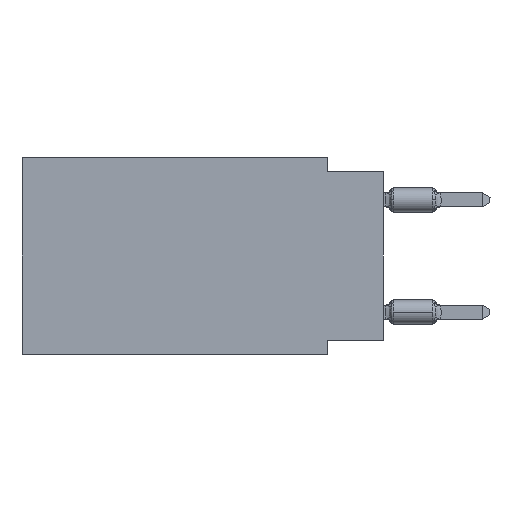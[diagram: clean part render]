
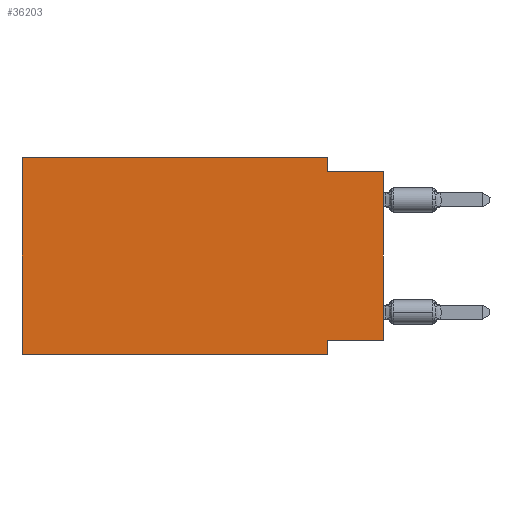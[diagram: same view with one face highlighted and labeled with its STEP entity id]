
A CAD part, left-side view. The second image highlights one B-rep face of the part: STEP entity #36203.
In plain terms, the highlighted planar face has unit normal (-1, 0, 0).
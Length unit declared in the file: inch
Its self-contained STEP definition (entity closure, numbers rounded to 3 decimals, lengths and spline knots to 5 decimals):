
#1443 = VERTEX_POINT ( 'NONE', #53261 ) ;
#1887 = ORIENTED_EDGE ( 'NONE', *, *, #59351, .F. ) ;
#2202 = CARTESIAN_POINT ( 'NONE',  ( 0., 0.645, -0.35 ) ) ;
#2597 = CARTESIAN_POINT ( 'NONE',  ( 0., 0., 0. ) ) ;
#3187 = VECTOR ( 'NONE', #30188, 39.37008 ) ;
#3581 = ORIENTED_EDGE ( 'NONE', *, *, #48791, .F. ) ;
#4973 = DIRECTION ( 'NONE',  ( 0., 0., 1. ) ) ;
#5884 = LINE ( 'NONE', #10403, #34656 ) ;
#6869 = CARTESIAN_POINT ( 'NONE',  ( 0., 0.645, 0. ) ) ;
#6891 = VECTOR ( 'NONE', #37320, 39.37008 ) ;
#8120 = VECTOR ( 'NONE', #14728, 39.37008 ) ;
#9150 = EDGE_CURVE ( 'NONE', #45152, #1443, #17532, .T. ) ;
#9815 = VECTOR ( 'NONE', #4973, 39.37008 ) ;
#10074 = CARTESIAN_POINT ( 'NONE',  ( 0., 0.1, -0.025 ) ) ;
#10147 = CARTESIAN_POINT ( 'NONE',  ( 0., 0.645, 0. ) ) ;
#10403 = CARTESIAN_POINT ( 'NONE',  ( 0., 0.645, -0.35 ) ) ;
#11067 = EDGE_CURVE ( 'NONE', #25647, #43677, #47389, .T. ) ;
#11736 = PLANE ( 'NONE',  #49026 ) ;
#14728 = DIRECTION ( 'NONE',  ( 0., 0., -1. ) ) ;
#15031 = LINE ( 'NONE', #10147, #9815 ) ;
#16442 = CARTESIAN_POINT ( 'NONE',  ( 0., 0., -0.325 ) ) ;
#17162 = VECTOR ( 'NONE', #35926, 39.37008 ) ;
#17532 = LINE ( 'NONE', #51068, #25359 ) ;
#22454 = ORIENTED_EDGE ( 'NONE', *, *, #25633, .F. ) ;
#22776 = ORIENTED_EDGE ( 'NONE', *, *, #9150, .F. ) ;
#24772 = CARTESIAN_POINT ( 'NONE',  ( 0., 0., -0.325 ) ) ;
#25254 = CARTESIAN_POINT ( 'NONE',  ( 0., 0., -0.025 ) ) ;
#25359 = VECTOR ( 'NONE', #25445, 39.37008 ) ;
#25445 = DIRECTION ( 'NONE',  ( 0., 0., -1. ) ) ;
#25633 = EDGE_CURVE ( 'NONE', #41551, #64042, #15031, .T. ) ;
#25647 = VERTEX_POINT ( 'NONE', #24772 ) ;
#26013 = VERTEX_POINT ( 'NONE', #10074 ) ;
#27082 = VECTOR ( 'NONE', #49104, 39.37008 ) ;
#30188 = DIRECTION ( 'NONE',  ( 0., -1., 0. ) ) ;
#33506 = ORIENTED_EDGE ( 'NONE', *, *, #38036, .T. ) ;
#34480 = CARTESIAN_POINT ( 'NONE',  ( 0., 0.645, 0. ) ) ;
#34656 = VECTOR ( 'NONE', #35402, 39.37008 ) ;
#34739 = EDGE_CURVE ( 'NONE', #64042, #49921, #39049, .T. ) ;
#34744 = LINE ( 'NONE', #49360, #3187 ) ;
#35402 = DIRECTION ( 'NONE',  ( 0., -1., 0. ) ) ;
#35744 = EDGE_LOOP ( 'NONE', ( #63016, #53160, #1887, #54728, #22454, #33506, #22776, #3581 ) ) ;
#35926 = DIRECTION ( 'NONE',  ( 0., 1., 0. ) ) ;
#36203 = ADVANCED_FACE ( 'NONE', ( #36402 ), #11736, .F. ) ;
#36402 = FACE_OUTER_BOUND ( 'NONE', #35744, .T. ) ;
#37320 = DIRECTION ( 'NONE',  ( 0., 0., 1. ) ) ;
#38036 = EDGE_CURVE ( 'NONE', #41551, #1443, #5884, .T. ) ;
#39049 = LINE ( 'NONE', #34480, #27082 ) ;
#41551 = VERTEX_POINT ( 'NONE', #2202 ) ;
#42492 = CARTESIAN_POINT ( 'NONE',  ( 0., 0.1, -0.325 ) ) ;
#43677 = VERTEX_POINT ( 'NONE', #25254 ) ;
#44287 = CARTESIAN_POINT ( 'NONE',  ( 0., 0.1, 0. ) ) ;
#44593 = LINE ( 'NONE', #44287, #8120 ) ;
#44711 = CARTESIAN_POINT ( 'NONE',  ( 0., 0.1, 0. ) ) ;
#45152 = VERTEX_POINT ( 'NONE', #42492 ) ;
#47114 = DIRECTION ( 'NONE',  ( 0., 0., -1. ) ) ;
#47389 = LINE ( 'NONE', #2597, #6891 ) ;
#48791 = EDGE_CURVE ( 'NONE', #25647, #45152, #56045, .T. ) ;
#49026 = AXIS2_PLACEMENT_3D ( 'NONE', #6869, #62049, #47114 ) ;
#49104 = DIRECTION ( 'NONE',  ( 0., -1., 0. ) ) ;
#49360 = CARTESIAN_POINT ( 'NONE',  ( 0., 0., -0.025 ) ) ;
#49921 = VERTEX_POINT ( 'NONE', #44711 ) ;
#51068 = CARTESIAN_POINT ( 'NONE',  ( 0., 0.1, -0.35 ) ) ;
#53160 = ORIENTED_EDGE ( 'NONE', *, *, #63951, .F. ) ;
#53261 = CARTESIAN_POINT ( 'NONE',  ( 0., 0.1, -0.35 ) ) ;
#54728 = ORIENTED_EDGE ( 'NONE', *, *, #34739, .F. ) ;
#56045 = LINE ( 'NONE', #16442, #17162 ) ;
#57100 = CARTESIAN_POINT ( 'NONE',  ( 0., 0.645, 0. ) ) ;
#59351 = EDGE_CURVE ( 'NONE', #49921, #26013, #44593, .T. ) ;
#62049 = DIRECTION ( 'NONE',  ( 1., 0., 0. ) ) ;
#63016 = ORIENTED_EDGE ( 'NONE', *, *, #11067, .T. ) ;
#63951 = EDGE_CURVE ( 'NONE', #26013, #43677, #34744, .T. ) ;
#64042 = VERTEX_POINT ( 'NONE', #57100 ) ;
